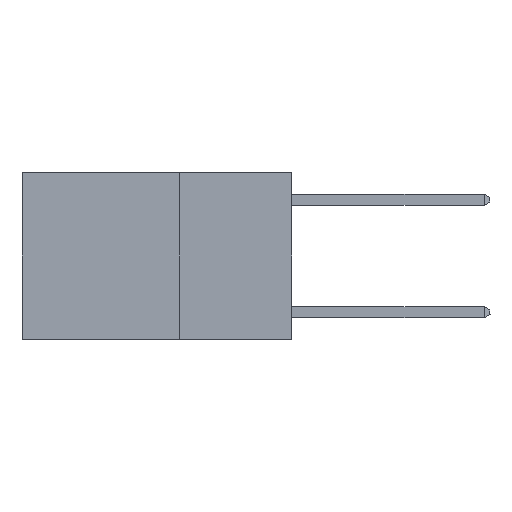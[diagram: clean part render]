
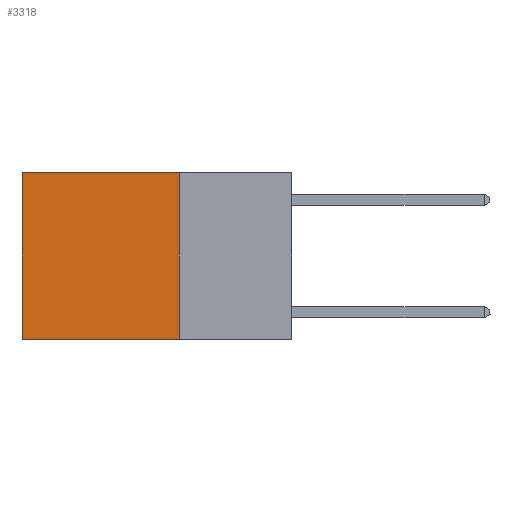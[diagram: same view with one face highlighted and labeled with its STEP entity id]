
A CAD part, left-side view. The second image highlights one B-rep face of the part: STEP entity #3318.
In plain terms, the highlighted planar face has unit normal (-1, 0, 0).
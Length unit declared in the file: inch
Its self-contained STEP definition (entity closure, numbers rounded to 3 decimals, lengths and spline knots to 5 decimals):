
#514 = ORIENTED_EDGE ( 'NONE', *, *, #10162, .T. ) ;
#1366 = EDGE_CURVE ( 'NONE', #14571, #15449, #18302, .T. ) ;
#1512 = DIRECTION ( 'NONE',  ( 0., 0., -1. ) ) ;
#1816 = CARTESIAN_POINT ( 'NONE',  ( 0.2625, 0.6, 0. ) ) ;
#1828 = ORIENTED_EDGE ( 'NONE', *, *, #12799, .F. ) ;
#2621 = FACE_OUTER_BOUND ( 'NONE', #12776, .T. ) ;
#3318 = ADVANCED_FACE ( 'NONE', ( #2621 ), #6592, .F. ) ;
#3439 = ORIENTED_EDGE ( 'NONE', *, *, #20323, .F. ) ;
#3526 = DIRECTION ( 'NONE',  ( 0., 0., -1. ) ) ;
#3649 = VERTEX_POINT ( 'NONE', #8008 ) ;
#3958 = ORIENTED_EDGE ( 'NONE', *, *, #1366, .T. ) ;
#4059 = CARTESIAN_POINT ( 'NONE',  ( 0.2625, 0.25, 0. ) ) ;
#6592 = PLANE ( 'NONE',  #20998 ) ;
#7699 = DIRECTION ( 'NONE',  ( 0., 1., 0. ) ) ;
#7713 = VECTOR ( 'NONE', #7699, 39.37008 ) ;
#8008 = CARTESIAN_POINT ( 'NONE',  ( 0.2625, 0.25, -0.37 ) ) ;
#9283 = CARTESIAN_POINT ( 'NONE',  ( 0.2625, 0.6, -0.37 ) ) ;
#10162 = EDGE_CURVE ( 'NONE', #21675, #14571, #21122, .T. ) ;
#11753 = DIRECTION ( 'NONE',  ( 1., 0., 0. ) ) ;
#12215 = VECTOR ( 'NONE', #19283, 39.37008 ) ;
#12601 = CARTESIAN_POINT ( 'NONE',  ( 0.2625, 0.25, -0.37 ) ) ;
#12758 = VECTOR ( 'NONE', #14338, 39.37008 ) ;
#12776 = EDGE_LOOP ( 'NONE', ( #3958, #3439, #1828, #514 ) ) ;
#12799 = EDGE_CURVE ( 'NONE', #21675, #3649, #16724, .T. ) ;
#14338 = DIRECTION ( 'NONE',  ( 0., 1., 0. ) ) ;
#14571 = VERTEX_POINT ( 'NONE', #18874 ) ;
#15449 = VERTEX_POINT ( 'NONE', #9283 ) ;
#16158 = CARTESIAN_POINT ( 'NONE',  ( 0.2625, 0.25, 0. ) ) ;
#16692 = CARTESIAN_POINT ( 'NONE',  ( 0.2625, 0.25, 0. ) ) ;
#16724 = LINE ( 'NONE', #4059, #12215 ) ;
#16806 = CARTESIAN_POINT ( 'NONE',  ( 0.2625, 0.25, 0. ) ) ;
#17808 = VECTOR ( 'NONE', #3526, 39.37008 ) ;
#18302 = LINE ( 'NONE', #1816, #17808 ) ;
#18874 = CARTESIAN_POINT ( 'NONE',  ( 0.2625, 0.6, 0. ) ) ;
#19283 = DIRECTION ( 'NONE',  ( 0., 0., -1. ) ) ;
#20323 = EDGE_CURVE ( 'NONE', #3649, #15449, #21623, .T. ) ;
#20998 = AXIS2_PLACEMENT_3D ( 'NONE', #16806, #11753, #1512 ) ;
#21122 = LINE ( 'NONE', #16158, #7713 ) ;
#21623 = LINE ( 'NONE', #12601, #12758 ) ;
#21675 = VERTEX_POINT ( 'NONE', #16692 ) ;
